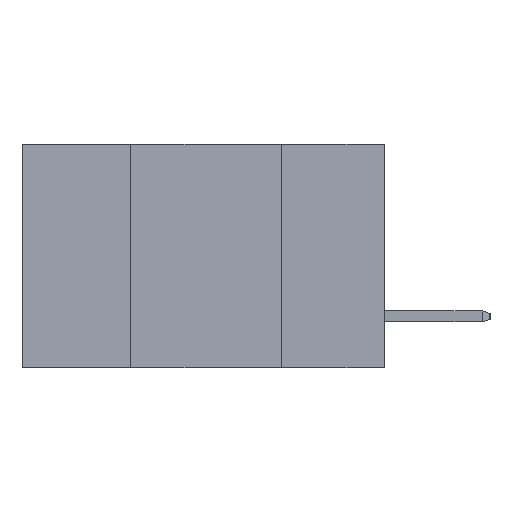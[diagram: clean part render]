
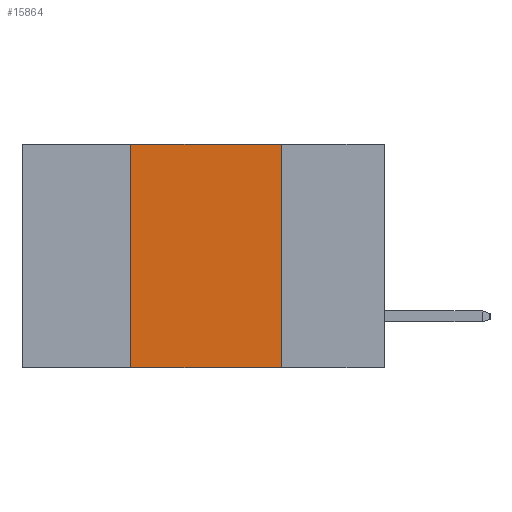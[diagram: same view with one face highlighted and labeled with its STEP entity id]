
A CAD part, left-side view. The second image highlights one B-rep face of the part: STEP entity #15864.
In plain terms, the highlighted planar face has unit normal (-1, 0, 0).
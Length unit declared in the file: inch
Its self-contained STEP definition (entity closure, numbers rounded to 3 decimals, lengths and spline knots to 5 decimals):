
#183 = EDGE_LOOP ( 'NONE', ( #10646, #400, #11409, #12760 ) ) ;
#400 = ORIENTED_EDGE ( 'NONE', *, *, #14328, .F. ) ;
#546 = PLANE ( 'NONE',  #13598 ) ;
#1079 = VERTEX_POINT ( 'NONE', #11157 ) ;
#1413 = FACE_OUTER_BOUND ( 'NONE', #183, .T. ) ;
#3430 = EDGE_CURVE ( 'NONE', #13554, #17599, #18034, .T. ) ;
#3719 = CARTESIAN_POINT ( 'NONE',  ( 0., 0.17, -0.37 ) ) ;
#5334 = CARTESIAN_POINT ( 'NONE',  ( 0., 0.42, 0. ) ) ;
#5442 = EDGE_CURVE ( 'NONE', #1079, #17644, #5597, .T. ) ;
#5597 = LINE ( 'NONE', #8915, #14067 ) ;
#6052 = CARTESIAN_POINT ( 'NONE',  ( 0., 0.6, 0. ) ) ;
#6168 = EDGE_CURVE ( 'NONE', #13554, #17644, #15177, .T. ) ;
#6171 = VECTOR ( 'NONE', #8438, 39.37008 ) ;
#6530 = CARTESIAN_POINT ( 'NONE',  ( 0., 0.42, -0.37 ) ) ;
#7903 = DIRECTION ( 'NONE',  ( 0., 0., -1. ) ) ;
#8438 = DIRECTION ( 'NONE',  ( 0., -1., 0. ) ) ;
#8442 = DIRECTION ( 'NONE',  ( 0., 0., -1. ) ) ;
#8516 = CARTESIAN_POINT ( 'NONE',  ( 0., 0.6, -0.37 ) ) ;
#8915 = CARTESIAN_POINT ( 'NONE',  ( 0., 0.17, -0.37 ) ) ;
#9105 = VECTOR ( 'NONE', #19180, 39.37008 ) ;
#10646 = ORIENTED_EDGE ( 'NONE', *, *, #5442, .F. ) ;
#11157 = CARTESIAN_POINT ( 'NONE',  ( 0., 0.17, 0. ) ) ;
#11409 = ORIENTED_EDGE ( 'NONE', *, *, #3430, .F. ) ;
#11963 = VECTOR ( 'NONE', #19285, 39.37008 ) ;
#12545 = LINE ( 'NONE', #17507, #11963 ) ;
#12760 = ORIENTED_EDGE ( 'NONE', *, *, #6168, .T. ) ;
#13554 = VERTEX_POINT ( 'NONE', #6530 ) ;
#13598 = AXIS2_PLACEMENT_3D ( 'NONE', #6052, #18616, #7903 ) ;
#14067 = VECTOR ( 'NONE', #8442, 39.37008 ) ;
#14328 = EDGE_CURVE ( 'NONE', #17599, #1079, #12545, .T. ) ;
#15177 = LINE ( 'NONE', #8516, #6171 ) ;
#15864 = ADVANCED_FACE ( 'NONE', ( #1413 ), #546, .F. ) ;
#17507 = CARTESIAN_POINT ( 'NONE',  ( 0., 0.6, 0. ) ) ;
#17599 = VERTEX_POINT ( 'NONE', #5334 ) ;
#17644 = VERTEX_POINT ( 'NONE', #3719 ) ;
#18034 = LINE ( 'NONE', #19207, #9105 ) ;
#18616 = DIRECTION ( 'NONE',  ( 1., 0., 0. ) ) ;
#19180 = DIRECTION ( 'NONE',  ( 0., 0., 1. ) ) ;
#19207 = CARTESIAN_POINT ( 'NONE',  ( 0., 0.42, -0.37 ) ) ;
#19285 = DIRECTION ( 'NONE',  ( 0., -1., 0. ) ) ;
